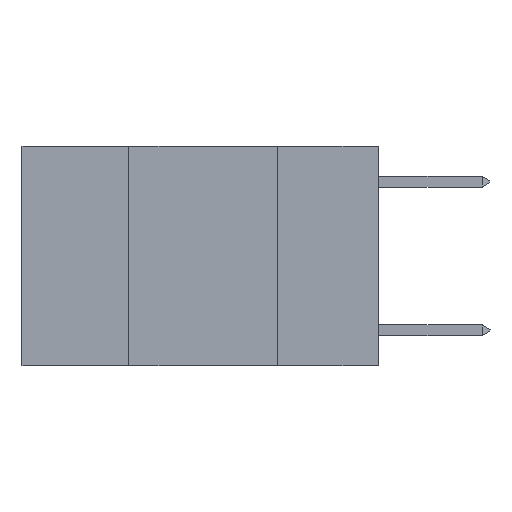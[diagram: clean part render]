
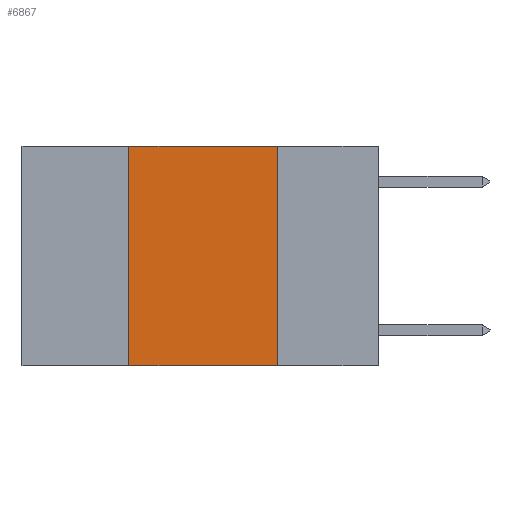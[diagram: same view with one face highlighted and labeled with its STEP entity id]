
A CAD part, left-side view. The second image highlights one B-rep face of the part: STEP entity #6867.
In plain terms, the highlighted planar face has unit normal (-1, 0, 0).
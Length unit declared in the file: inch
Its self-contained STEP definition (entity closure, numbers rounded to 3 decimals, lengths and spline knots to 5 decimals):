
#83 = FACE_OUTER_BOUND ( 'NONE', #11257, .T. ) ;
#215 = CARTESIAN_POINT ( 'NONE',  ( 0., 0.6, 0. ) ) ;
#1569 = LINE ( 'NONE', #1843, #16906 ) ;
#1843 = CARTESIAN_POINT ( 'NONE',  ( 0., 0.42, 0. ) ) ;
#2008 = DIRECTION ( 'NONE',  ( 0., -1., 0. ) ) ;
#2326 = VERTEX_POINT ( 'NONE', #18761 ) ;
#2358 = ORIENTED_EDGE ( 'NONE', *, *, #13116, .F. ) ;
#2819 = ORIENTED_EDGE ( 'NONE', *, *, #4754, .F. ) ;
#2883 = ORIENTED_EDGE ( 'NONE', *, *, #8732, .F. ) ;
#3528 = ORIENTED_EDGE ( 'NONE', *, *, #13151, .T. ) ;
#3784 = LINE ( 'NONE', #7272, #18092 ) ;
#4681 = PLANE ( 'NONE',  #8484 ) ;
#4754 = EDGE_CURVE ( 'NONE', #15836, #10554, #10347, .T. ) ;
#5687 = DIRECTION ( 'NONE',  ( 0., 0., -1. ) ) ;
#5762 = DIRECTION ( 'NONE',  ( 0., -1., 0. ) ) ;
#6867 = ADVANCED_FACE ( 'NONE', ( #83 ), #4681, .F. ) ;
#7272 = CARTESIAN_POINT ( 'NONE',  ( 0., 0.17, 0. ) ) ;
#7853 = DIRECTION ( 'NONE',  ( 1., 0., 0. ) ) ;
#8484 = AXIS2_PLACEMENT_3D ( 'NONE', #215, #7853, #17956 ) ;
#8732 = EDGE_CURVE ( 'NONE', #17177, #15836, #1569, .T. ) ;
#10154 = CARTESIAN_POINT ( 'NONE',  ( 0., 0.42, -0.37 ) ) ;
#10297 = CARTESIAN_POINT ( 'NONE',  ( 0., 0.6, -0.37 ) ) ;
#10347 = LINE ( 'NONE', #16891, #13212 ) ;
#10554 = VERTEX_POINT ( 'NONE', #18202 ) ;
#11257 = EDGE_LOOP ( 'NONE', ( #2358, #2819, #2883, #3528 ) ) ;
#12350 = DIRECTION ( 'NONE',  ( 0., 0., 1. ) ) ;
#13116 = EDGE_CURVE ( 'NONE', #10554, #2326, #3784, .T. ) ;
#13151 = EDGE_CURVE ( 'NONE', #17177, #2326, #14304, .T. ) ;
#13212 = VECTOR ( 'NONE', #2008, 39.37008 ) ;
#13851 = CARTESIAN_POINT ( 'NONE',  ( 0., 0.42, 0. ) ) ;
#14304 = LINE ( 'NONE', #10297, #17663 ) ;
#15836 = VERTEX_POINT ( 'NONE', #13851 ) ;
#16891 = CARTESIAN_POINT ( 'NONE',  ( 0., 0.6, 0. ) ) ;
#16906 = VECTOR ( 'NONE', #12350, 39.37008 ) ;
#17177 = VERTEX_POINT ( 'NONE', #10154 ) ;
#17663 = VECTOR ( 'NONE', #5762, 39.37008 ) ;
#17956 = DIRECTION ( 'NONE',  ( 0., 0., -1. ) ) ;
#18092 = VECTOR ( 'NONE', #5687, 39.37008 ) ;
#18202 = CARTESIAN_POINT ( 'NONE',  ( 0., 0.17, 0. ) ) ;
#18761 = CARTESIAN_POINT ( 'NONE',  ( 0., 0.17, -0.37 ) ) ;
